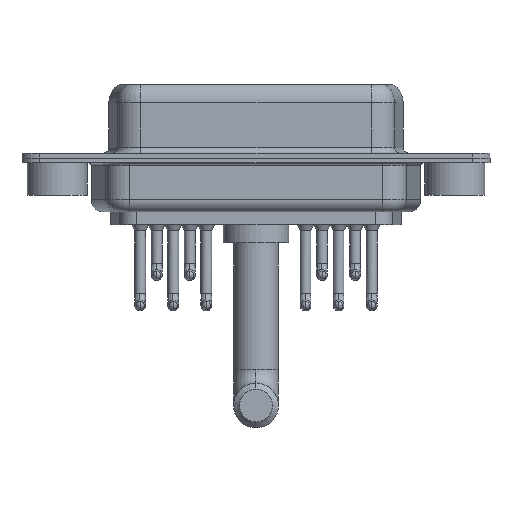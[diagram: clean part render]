
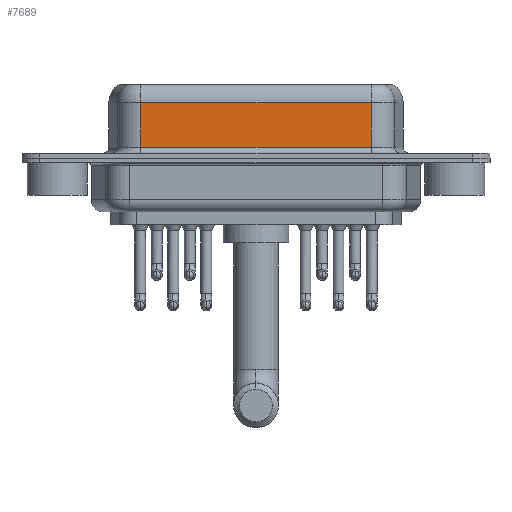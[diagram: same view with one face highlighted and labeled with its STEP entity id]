
A CAD part, front view. The second image highlights one B-rep face of the part: STEP entity #7689.
In plain terms, the highlighted planar face has unit normal (0, -1, 0).
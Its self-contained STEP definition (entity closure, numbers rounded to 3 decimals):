
#1121 = AXIS2_PLACEMENT_3D ( 'NONE', #9526, #15293, #6480 ) ;
#1717 = VECTOR ( 'NONE', #13479, 1000. ) ;
#1901 = PLANE ( 'NONE',  #1121 ) ;
#2100 = VECTOR ( 'NONE', #12400, 1000. ) ;
#2381 = VERTEX_POINT ( 'NONE', #8614 ) ;
#2942 = VERTEX_POINT ( 'NONE', #16030 ) ;
#6480 = DIRECTION ( 'NONE',  ( 0., 0., 1. ) ) ;
#6675 = EDGE_LOOP ( 'NONE', ( #10894, #18499, #13750, #14680 ) ) ;
#7020 = EDGE_CURVE ( 'NONE', #2942, #2381, #8600, .T. ) ;
#7207 = LINE ( 'NONE', #15910, #8511 ) ;
#7689 = ADVANCED_FACE ( 'NONE', ( #13710 ), #1901, .F. ) ;
#8511 = VECTOR ( 'NONE', #16000, 1000. ) ;
#8600 = LINE ( 'NONE', #12579, #10513 ) ;
#8614 = CARTESIAN_POINT ( 'NONE',  ( 7.013, -3.95, 4.65 ) ) ;
#9380 = VERTEX_POINT ( 'NONE', #10679 ) ;
#9526 = CARTESIAN_POINT ( 'NONE',  ( 26.287, -3.95, 6.4 ) ) ;
#9828 = DIRECTION ( 'NONE',  ( -1., 0., 0. ) ) ;
#10176 = EDGE_CURVE ( 'NONE', #2381, #9380, #7207, .T. ) ;
#10513 = VECTOR ( 'NONE', #9828, 1000. ) ;
#10679 = CARTESIAN_POINT ( 'NONE',  ( 7.013, -3.95, 0.9 ) ) ;
#10894 = ORIENTED_EDGE ( 'NONE', *, *, #16130, .F. ) ;
#12400 = DIRECTION ( 'NONE',  ( 0., 0., -1. ) ) ;
#12495 = CARTESIAN_POINT ( 'NONE',  ( 26.287, -3.95, 6.4 ) ) ;
#12579 = CARTESIAN_POINT ( 'NONE',  ( 26.287, -3.95, 4.65 ) ) ;
#12930 = CARTESIAN_POINT ( 'NONE',  ( 26.287, -3.95, 0.9 ) ) ;
#13479 = DIRECTION ( 'NONE',  ( 1., 0., 0. ) ) ;
#13569 = LINE ( 'NONE', #17686, #1717 ) ;
#13710 = FACE_OUTER_BOUND ( 'NONE', #6675, .T. ) ;
#13727 = EDGE_CURVE ( 'NONE', #9380, #14870, #13569, .T. ) ;
#13750 = ORIENTED_EDGE ( 'NONE', *, *, #10176, .T. ) ;
#14680 = ORIENTED_EDGE ( 'NONE', *, *, #13727, .T. ) ;
#14870 = VERTEX_POINT ( 'NONE', #12930 ) ;
#15293 = DIRECTION ( 'NONE',  ( 0., 1., 0. ) ) ;
#15509 = LINE ( 'NONE', #12495, #2100 ) ;
#15910 = CARTESIAN_POINT ( 'NONE',  ( 7.013, -3.95, 6.4 ) ) ;
#16000 = DIRECTION ( 'NONE',  ( 0., 0., -1. ) ) ;
#16030 = CARTESIAN_POINT ( 'NONE',  ( 26.287, -3.95, 4.65 ) ) ;
#16130 = EDGE_CURVE ( 'NONE', #2942, #14870, #15509, .T. ) ;
#17686 = CARTESIAN_POINT ( 'NONE',  ( 26.287, -3.95, 0.9 ) ) ;
#18499 = ORIENTED_EDGE ( 'NONE', *, *, #7020, .T. ) ;
